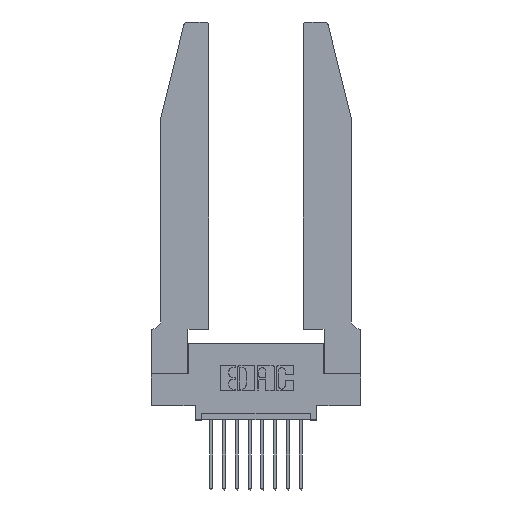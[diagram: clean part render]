
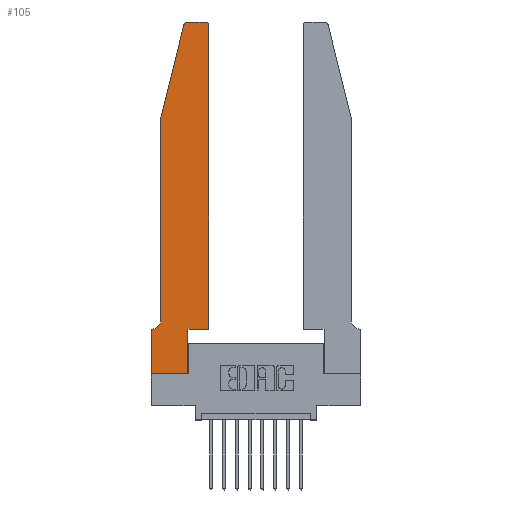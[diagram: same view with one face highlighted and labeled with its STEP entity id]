
A CAD part, top view. The second image highlights one B-rep face of the part: STEP entity #105.
In plain terms, the highlighted planar face has unit normal (0, 0, 1).
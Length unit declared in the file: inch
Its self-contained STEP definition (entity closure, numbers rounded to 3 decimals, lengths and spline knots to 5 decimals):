
#105 = ADVANCED_FACE ( 'NONE', ( #15265 ), #10515, .T. ) ;
#242 = VECTOR ( 'NONE', #586, 39.37008 ) ;
#311 = AXIS2_PLACEMENT_3D ( 'NONE', #10846, #1402, #4935 ) ;
#431 = AXIS2_PLACEMENT_3D ( 'NONE', #13102, #14801, #7315 ) ;
#586 = DIRECTION ( 'NONE',  ( 0., -1., 0. ) ) ;
#598 = VECTOR ( 'NONE', #8886, 39.37008 ) ;
#740 = VECTOR ( 'NONE', #9140, 39.37008 ) ;
#870 = VERTEX_POINT ( 'NONE', #9173 ) ;
#943 = CIRCLE ( 'NONE', #2707, 0.03 ) ;
#1000 = VERTEX_POINT ( 'NONE', #4982 ) ;
#1402 = DIRECTION ( 'NONE',  ( 0., 0., 1. ) ) ;
#1422 = CARTESIAN_POINT ( 'NONE',  ( 0.4505, 0.35, 0.37 ) ) ;
#2004 = ORIENTED_EDGE ( 'NONE', *, *, #13689, .T. ) ;
#2031 = VERTEX_POINT ( 'NONE', #6402 ) ;
#2158 = EDGE_CURVE ( 'NONE', #14990, #11135, #7890, .T. ) ;
#2163 = CARTESIAN_POINT ( 'NONE',  ( 0., 0.35, 0.37 ) ) ;
#2213 = CARTESIAN_POINT ( 'NONE',  ( 0., 0.35, 0.37 ) ) ;
#2399 = LINE ( 'NONE', #8625, #7073 ) ;
#2584 = CARTESIAN_POINT ( 'NONE',  ( 0., 0., 0.37 ) ) ;
#2707 = AXIS2_PLACEMENT_3D ( 'NONE', #5665, #10417, #11841 ) ;
#2711 = EDGE_CURVE ( 'NONE', #8139, #6229, #5272, .T. ) ;
#2755 = EDGE_CURVE ( 'NONE', #1000, #4954, #943, .T. ) ;
#3095 = ORIENTED_EDGE ( 'NONE', *, *, #3746, .T. ) ;
#3139 = VERTEX_POINT ( 'NONE', #6106 ) ;
#3233 = CARTESIAN_POINT ( 'NONE',  ( 0.284, 2.75, 0.37 ) ) ;
#3575 = CARTESIAN_POINT ( 'NONE',  ( 0.0755, 2., 0.37 ) ) ;
#3746 = EDGE_CURVE ( 'NONE', #5573, #8139, #5601, .T. ) ;
#3841 = CARTESIAN_POINT ( 'NONE',  ( 0.4205, 2.75, 0.37 ) ) ;
#3977 = VECTOR ( 'NONE', #8036, 39.37008 ) ;
#4139 = EDGE_CURVE ( 'NONE', #13162, #7639, #7259, .T. ) ;
#4174 = LINE ( 'NONE', #10124, #15220 ) ;
#4382 = CARTESIAN_POINT ( 'NONE',  ( 0.25487, 2.72718, 0.37 ) ) ;
#4397 = CARTESIAN_POINT ( 'NONE',  ( 0.0755, 2., 0.37 ) ) ;
#4567 = ORIENTED_EDGE ( 'NONE', *, *, #2755, .T. ) ;
#4732 = ORIENTED_EDGE ( 'NONE', *, *, #2158, .T. ) ;
#4935 = DIRECTION ( 'NONE',  ( 1., 0., 0. ) ) ;
#4954 = VERTEX_POINT ( 'NONE', #3841 ) ;
#4982 = CARTESIAN_POINT ( 'NONE',  ( 0.4505, 2.72, 0.37 ) ) ;
#4999 = ORIENTED_EDGE ( 'NONE', *, *, #10074, .T. ) ;
#5272 = LINE ( 'NONE', #11326, #598 ) ;
#5573 = VERTEX_POINT ( 'NONE', #3233 ) ;
#5601 = CIRCLE ( 'NONE', #311, 0.03 ) ;
#5665 = CARTESIAN_POINT ( 'NONE',  ( 0.4205, 2.72, 0.37 ) ) ;
#5883 = DIRECTION ( 'NONE',  ( 1., 0., 0. ) ) ;
#5988 = CARTESIAN_POINT ( 'NONE',  ( 0., 0., 0.37 ) ) ;
#6106 = CARTESIAN_POINT ( 'NONE',  ( 0.2865, 0., 0.37 ) ) ;
#6229 = VERTEX_POINT ( 'NONE', #3575 ) ;
#6312 = ORIENTED_EDGE ( 'NONE', *, *, #13403, .T. ) ;
#6402 = CARTESIAN_POINT ( 'NONE',  ( 0.4505, 0.35, 0.37 ) ) ;
#6428 = ORIENTED_EDGE ( 'NONE', *, *, #9473, .T. ) ;
#7012 = DIRECTION ( 'NONE',  ( 1., 0., 0. ) ) ;
#7073 = VECTOR ( 'NONE', #12378, 39.37008 ) ;
#7259 = CIRCLE ( 'NONE', #431, 0.07 ) ;
#7315 = DIRECTION ( 'NONE',  ( -1., 0., 0. ) ) ;
#7489 = DIRECTION ( 'NONE',  ( 0., 1., 0. ) ) ;
#7639 = VERTEX_POINT ( 'NONE', #8616 ) ;
#7729 = LINE ( 'NONE', #4397, #3977 ) ;
#7816 = DIRECTION ( 'NONE',  ( -1., 0., 0. ) ) ;
#7857 = EDGE_CURVE ( 'NONE', #6229, #13162, #7729, .T. ) ;
#7890 = LINE ( 'NONE', #12447, #242 ) ;
#8036 = DIRECTION ( 'NONE',  ( 0., -1., 0. ) ) ;
#8139 = VERTEX_POINT ( 'NONE', #4382 ) ;
#8379 = ORIENTED_EDGE ( 'NONE', *, *, #15139, .T. ) ;
#8616 = CARTESIAN_POINT ( 'NONE',  ( 0.0055, 0.35, 0.37 ) ) ;
#8625 = CARTESIAN_POINT ( 'NONE',  ( 0.2605, 2.75, 0.37 ) ) ;
#8886 = DIRECTION ( 'NONE',  ( -0.239, -0.971, 0. ) ) ;
#9140 = DIRECTION ( 'NONE',  ( 0., 1., 0. ) ) ;
#9173 = CARTESIAN_POINT ( 'NONE',  ( 0.2865, 0.35, 0.37 ) ) ;
#9473 = EDGE_CURVE ( 'NONE', #3139, #870, #10980, .T. ) ;
#9947 = ORIENTED_EDGE ( 'NONE', *, *, #2711, .T. ) ;
#10038 = CARTESIAN_POINT ( 'NONE',  ( 0.2865, 0.35, 0.37 ) ) ;
#10074 = EDGE_CURVE ( 'NONE', #2031, #1000, #13803, .T. ) ;
#10124 = CARTESIAN_POINT ( 'NONE',  ( 0.0755, 0.35, 0.37 ) ) ;
#10199 = VECTOR ( 'NONE', #7489, 39.37008 ) ;
#10417 = DIRECTION ( 'NONE',  ( 0., 0., 1. ) ) ;
#10515 = PLANE ( 'NONE',  #11543 ) ;
#10586 = VECTOR ( 'NONE', #5883, 39.37008 ) ;
#10772 = ORIENTED_EDGE ( 'NONE', *, *, #11499, .T. ) ;
#10846 = CARTESIAN_POINT ( 'NONE',  ( 0.284, 2.72, 0.37 ) ) ;
#10980 = LINE ( 'NONE', #10038, #740 ) ;
#11135 = VERTEX_POINT ( 'NONE', #2584 ) ;
#11326 = CARTESIAN_POINT ( 'NONE',  ( 0.0755, 2., 0.37 ) ) ;
#11499 = EDGE_CURVE ( 'NONE', #7639, #14990, #4174, .T. ) ;
#11533 = LINE ( 'NONE', #14130, #10586 ) ;
#11543 = AXIS2_PLACEMENT_3D ( 'NONE', #2163, #15446, #7012 ) ;
#11841 = DIRECTION ( 'NONE',  ( 1., 0., 0. ) ) ;
#11865 = ORIENTED_EDGE ( 'NONE', *, *, #7857, .T. ) ;
#12378 = DIRECTION ( 'NONE',  ( -1., 0., 0. ) ) ;
#12447 = CARTESIAN_POINT ( 'NONE',  ( 0., 0., 0.37 ) ) ;
#12488 = CARTESIAN_POINT ( 'NONE',  ( 0.0755, 0.42, 0.37 ) ) ;
#12645 = ORIENTED_EDGE ( 'NONE', *, *, #4139, .T. ) ;
#13102 = CARTESIAN_POINT ( 'NONE',  ( 0.0055, 0.42, 0.37 ) ) ;
#13162 = VERTEX_POINT ( 'NONE', #12488 ) ;
#13167 = EDGE_LOOP ( 'NONE', ( #2004, #3095, #9947, #11865, #12645, #10772, #4732, #8379, #6428, #6312, #4999, #4567 ) ) ;
#13403 = EDGE_CURVE ( 'NONE', #870, #2031, #11533, .T. ) ;
#13689 = EDGE_CURVE ( 'NONE', #4954, #5573, #2399, .T. ) ;
#13803 = LINE ( 'NONE', #1422, #10199 ) ;
#14130 = CARTESIAN_POINT ( 'NONE',  ( 0.4505, 0.35, 0.37 ) ) ;
#14332 = DIRECTION ( 'NONE',  ( 1., 0., 0. ) ) ;
#14801 = DIRECTION ( 'NONE',  ( 0., 0., -1. ) ) ;
#14990 = VERTEX_POINT ( 'NONE', #2213 ) ;
#15139 = EDGE_CURVE ( 'NONE', #11135, #3139, #15407, .T. ) ;
#15220 = VECTOR ( 'NONE', #7816, 39.37008 ) ;
#15221 = VECTOR ( 'NONE', #14332, 39.37008 ) ;
#15265 = FACE_OUTER_BOUND ( 'NONE', #13167, .T. ) ;
#15407 = LINE ( 'NONE', #5988, #15221 ) ;
#15446 = DIRECTION ( 'NONE',  ( 0., 0., 1. ) ) ;
